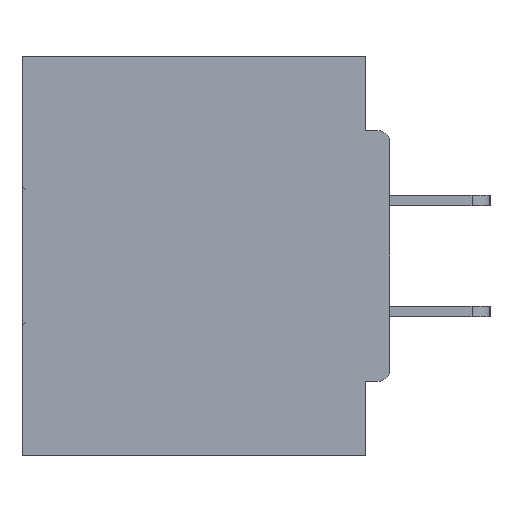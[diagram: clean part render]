
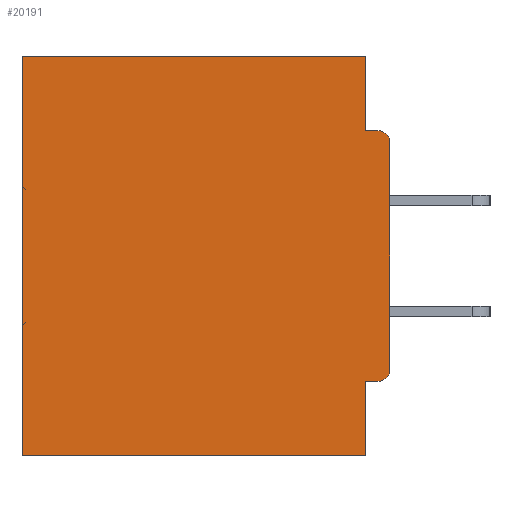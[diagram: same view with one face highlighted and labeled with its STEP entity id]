
A CAD part, left-side view. The second image highlights one B-rep face of the part: STEP entity #20191.
In plain terms, the highlighted planar face has unit normal (-1, 0, 0).
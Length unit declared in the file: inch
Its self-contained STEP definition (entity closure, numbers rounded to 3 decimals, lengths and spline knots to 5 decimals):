
#188 = DIRECTION ( 'NONE',  ( 1., 0., 0. ) ) ;
#837 = CARTESIAN_POINT ( 'NONE',  ( 0.298, 0., -0.0935 ) ) ;
#1069 = LINE ( 'NONE', #837, #3278 ) ;
#1192 = VERTEX_POINT ( 'NONE', #40722 ) ;
#1661 = VECTOR ( 'NONE', #22234, 39.37008 ) ;
#1948 = DIRECTION ( 'NONE',  ( 0., 0., -1. ) ) ;
#2235 = CIRCLE ( 'NONE', #24085, 0.015 ) ;
#2608 = EDGE_CURVE ( 'NONE', #18177, #9336, #2235, .T. ) ;
#3023 = VECTOR ( 'NONE', #31052, 39.37008 ) ;
#3278 = VECTOR ( 'NONE', #11116, 39.37008 ) ;
#3385 = ORIENTED_EDGE ( 'NONE', *, *, #17870, .F. ) ;
#4036 = LINE ( 'NONE', #40930, #30147 ) ;
#4191 = ORIENTED_EDGE ( 'NONE', *, *, #40619, .F. ) ;
#5704 = CARTESIAN_POINT ( 'NONE',  ( 0.298, 0.46, -0.5 ) ) ;
#5781 = DIRECTION ( 'NONE',  ( -1., 0., 0. ) ) ;
#6752 = VERTEX_POINT ( 'NONE', #13588 ) ;
#7791 = CARTESIAN_POINT ( 'NONE',  ( 0.298, 0.031, -0.5 ) ) ;
#8195 = ORIENTED_EDGE ( 'NONE', *, *, #41448, .F. ) ;
#8767 = CARTESIAN_POINT ( 'NONE',  ( 0.298, 0.46, 0. ) ) ;
#9336 = VERTEX_POINT ( 'NONE', #39449 ) ;
#10588 = CARTESIAN_POINT ( 'NONE',  ( 0.298, 0., -0.4065 ) ) ;
#11109 = AXIS2_PLACEMENT_3D ( 'NONE', #20842, #188, #24208 ) ;
#11116 = DIRECTION ( 'NONE',  ( 0., -1., 0. ) ) ;
#11276 = CARTESIAN_POINT ( 'NONE',  ( 0.298, 0., 0. ) ) ;
#11550 = EDGE_CURVE ( 'NONE', #1192, #35200, #33582, .T. ) ;
#12101 = LINE ( 'NONE', #40073, #38777 ) ;
#12474 = EDGE_CURVE ( 'NONE', #15916, #1192, #13291, .T. ) ;
#13200 = VERTEX_POINT ( 'NONE', #7791 ) ;
#13291 = LINE ( 'NONE', #20714, #3023 ) ;
#13588 = CARTESIAN_POINT ( 'NONE',  ( 0.298, 0.031, -0.4065 ) ) ;
#13610 = ORIENTED_EDGE ( 'NONE', *, *, #11550, .T. ) ;
#13893 = DIRECTION ( 'NONE',  ( 0., 1., 0. ) ) ;
#14295 = ORIENTED_EDGE ( 'NONE', *, *, #2608, .T. ) ;
#15429 = VERTEX_POINT ( 'NONE', #26197 ) ;
#15916 = VERTEX_POINT ( 'NONE', #27762 ) ;
#16951 = AXIS2_PLACEMENT_3D ( 'NONE', #43933, #5781, #20895 ) ;
#17798 = ORIENTED_EDGE ( 'NONE', *, *, #30886, .F. ) ;
#17870 = EDGE_CURVE ( 'NONE', #42015, #15429, #1069, .T. ) ;
#18177 = VERTEX_POINT ( 'NONE', #33234 ) ;
#19312 = CARTESIAN_POINT ( 'NONE',  ( 0.298, 0., -0.1085 ) ) ;
#19874 = VECTOR ( 'NONE', #28226, 39.37008 ) ;
#20191 = ADVANCED_FACE ( 'NONE', ( #34036 ), #28136, .F. ) ;
#20714 = CARTESIAN_POINT ( 'NONE',  ( 0.298, 0., 0. ) ) ;
#20744 = DIRECTION ( 'NONE',  ( 0., 0., -1. ) ) ;
#20842 = CARTESIAN_POINT ( 'NONE',  ( 0.298, 0., 0. ) ) ;
#20895 = DIRECTION ( 'NONE',  ( 0., 0., -1. ) ) ;
#21068 = VECTOR ( 'NONE', #13893, 39.37008 ) ;
#22088 = VERTEX_POINT ( 'NONE', #19312 ) ;
#22234 = DIRECTION ( 'NONE',  ( 0., 0., -1. ) ) ;
#22804 = ORIENTED_EDGE ( 'NONE', *, *, #30132, .F. ) ;
#24077 = EDGE_CURVE ( 'NONE', #22088, #9336, #29332, .T. ) ;
#24085 = AXIS2_PLACEMENT_3D ( 'NONE', #37657, #31083, #20744 ) ;
#24208 = DIRECTION ( 'NONE',  ( 0., 0., -1. ) ) ;
#25808 = CARTESIAN_POINT ( 'NONE',  ( 0.298, 0.031, -0.0935 ) ) ;
#26197 = CARTESIAN_POINT ( 'NONE',  ( 0.298, 0.015, -0.0935 ) ) ;
#26936 = ORIENTED_EDGE ( 'NONE', *, *, #44196, .T. ) ;
#27206 = DIRECTION ( 'NONE',  ( 0., 0., -1. ) ) ;
#27762 = CARTESIAN_POINT ( 'NONE',  ( 0.298, 0.031, 0. ) ) ;
#28136 = PLANE ( 'NONE',  #11109 ) ;
#28226 = DIRECTION ( 'NONE',  ( 0., 1., 0. ) ) ;
#29332 = LINE ( 'NONE', #11276, #1661 ) ;
#29373 = ORIENTED_EDGE ( 'NONE', *, *, #24077, .F. ) ;
#30132 = EDGE_CURVE ( 'NONE', #13200, #35200, #42854, .T. ) ;
#30147 = VECTOR ( 'NONE', #27206, 39.37008 ) ;
#30793 = CARTESIAN_POINT ( 'NONE',  ( 0.298, 0., -0.5 ) ) ;
#30886 = EDGE_CURVE ( 'NONE', #18177, #6752, #38384, .T. ) ;
#31052 = DIRECTION ( 'NONE',  ( 0., 1., 0. ) ) ;
#31083 = DIRECTION ( 'NONE',  ( -1., 0., 0. ) ) ;
#32801 = EDGE_LOOP ( 'NONE', ( #26936, #3385, #4191, #35745, #13610, #22804, #8195, #17798, #14295, #29373 ) ) ;
#33234 = CARTESIAN_POINT ( 'NONE',  ( 0.298, 0.015, -0.4065 ) ) ;
#33390 = DIRECTION ( 'NONE',  ( 0., 0., -1. ) ) ;
#33582 = LINE ( 'NONE', #8767, #40097 ) ;
#34036 = FACE_OUTER_BOUND ( 'NONE', #32801, .T. ) ;
#35101 = CIRCLE ( 'NONE', #16951, 0.015 ) ;
#35200 = VERTEX_POINT ( 'NONE', #5704 ) ;
#35745 = ORIENTED_EDGE ( 'NONE', *, *, #12474, .T. ) ;
#37657 = CARTESIAN_POINT ( 'NONE',  ( 0.298, 0.015, -0.3915 ) ) ;
#38384 = LINE ( 'NONE', #10588, #19874 ) ;
#38777 = VECTOR ( 'NONE', #33390, 39.37008 ) ;
#39449 = CARTESIAN_POINT ( 'NONE',  ( 0.298, 0., -0.3915 ) ) ;
#40073 = CARTESIAN_POINT ( 'NONE',  ( 0.298, 0.031, -0.5 ) ) ;
#40097 = VECTOR ( 'NONE', #1948, 39.37008 ) ;
#40619 = EDGE_CURVE ( 'NONE', #15916, #42015, #4036, .T. ) ;
#40722 = CARTESIAN_POINT ( 'NONE',  ( 0.298, 0.46, 0. ) ) ;
#40930 = CARTESIAN_POINT ( 'NONE',  ( 0.298, 0.031, -0.5 ) ) ;
#41448 = EDGE_CURVE ( 'NONE', #6752, #13200, #12101, .T. ) ;
#42015 = VERTEX_POINT ( 'NONE', #25808 ) ;
#42854 = LINE ( 'NONE', #30793, #21068 ) ;
#43933 = CARTESIAN_POINT ( 'NONE',  ( 0.298, 0.015, -0.1085 ) ) ;
#44196 = EDGE_CURVE ( 'NONE', #22088, #15429, #35101, .T. ) ;
